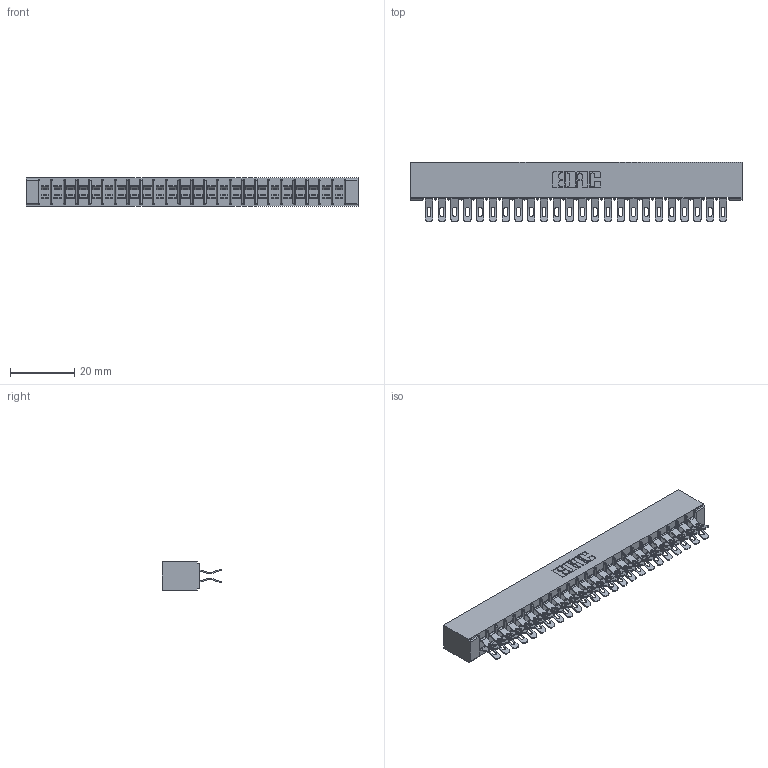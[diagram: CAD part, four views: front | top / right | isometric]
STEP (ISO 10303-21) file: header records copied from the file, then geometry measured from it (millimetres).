
FILE_DESCRIPTION (( 'STEP AP203' ), '1' );
FILE_NAME ('355-048-555-201.STEP', '2019-09-11T15:20:54', ( '' ), ( '' ), 'SwSTEP 2.0', 'SolidWorks 2016', '' );
FILE_SCHEMA (( 'CONFIG_CONTROL_DESIGN' ));
Length unit declared in the file: inch
Products named in the file (3): 305 Part_No Mounting; 355-048-555-201; 305-290-001_555
Assembly tree (49 placements, depth 2):
  355-048-555-201
    305 Part_No Mounting
    305-290-001_555  x48
Bounding box: 102.97 x 18.41 x 8.71 mm (x, y, z)
Volume: 6783.5 mm3; surface area: 14316.8 mm2
Topology: 49 solids, 49 shells, 3276 faces, 9772 edges, 6384 vertices
Faces by surface type: plane 1600, cylinder 1580, sphere 96
Entity records: 28523 total; most frequent: CARTESIAN_POINT 4736, ORIENTED_EDGE 4688, DIRECTION 4588, EDGE_CURVE 2344, LINE 1860, VECTOR 1860, VERTEX_POINT 1496, AXIS2_PLACEMENT_3D 1364
